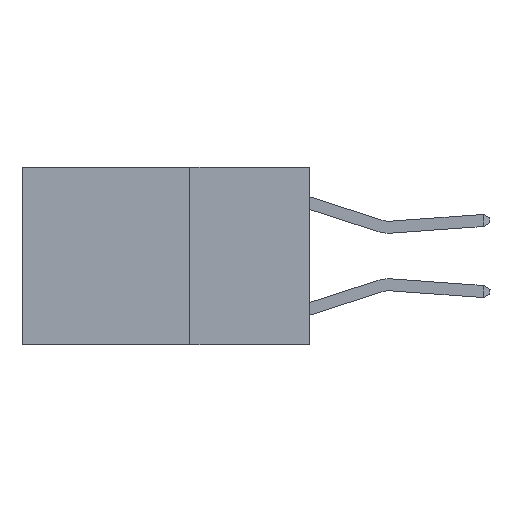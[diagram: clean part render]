
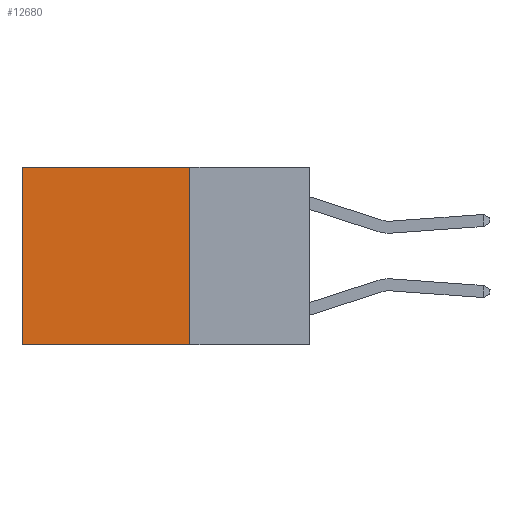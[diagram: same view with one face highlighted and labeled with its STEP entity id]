
A CAD part, left-side view. The second image highlights one B-rep face of the part: STEP entity #12680.
In plain terms, the highlighted planar face has unit normal (-1, 0, 0).
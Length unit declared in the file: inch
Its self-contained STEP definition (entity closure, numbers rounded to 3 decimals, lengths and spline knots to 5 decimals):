
#851 = LINE ( 'NONE', #23204, #16633 ) ;
#1499 = LINE ( 'NONE', #9269, #6930 ) ;
#1567 = ORIENTED_EDGE ( 'NONE', *, *, #6776, .T. ) ;
#1886 = ORIENTED_EDGE ( 'NONE', *, *, #24794, .F. ) ;
#3127 = VERTEX_POINT ( 'NONE', #9824 ) ;
#4340 = LINE ( 'NONE', #23465, #25507 ) ;
#4386 = EDGE_LOOP ( 'NONE', ( #1567, #4631, #1886, #12244 ) ) ;
#4631 = ORIENTED_EDGE ( 'NONE', *, *, #9931, .F. ) ;
#5051 = DIRECTION ( 'NONE',  ( 0., 0., -1. ) ) ;
#6243 = VERTEX_POINT ( 'NONE', #25667 ) ;
#6776 = EDGE_CURVE ( 'NONE', #3127, #23421, #851, .T. ) ;
#6930 = VECTOR ( 'NONE', #25627, 39.37008 ) ;
#9120 = CARTESIAN_POINT ( 'NONE',  ( 0.2625, 0.25, 0. ) ) ;
#9269 = CARTESIAN_POINT ( 'NONE',  ( 0.2625, 0.25, -0.37 ) ) ;
#9277 = CARTESIAN_POINT ( 'NONE',  ( 0.2625, 0.25, 0. ) ) ;
#9824 = CARTESIAN_POINT ( 'NONE',  ( 0.2625, 0.6, 0. ) ) ;
#9931 = EDGE_CURVE ( 'NONE', #19159, #23421, #1499, .T. ) ;
#11525 = EDGE_CURVE ( 'NONE', #6243, #3127, #24166, .T. ) ;
#12244 = ORIENTED_EDGE ( 'NONE', *, *, #11525, .T. ) ;
#12680 = ADVANCED_FACE ( 'NONE', ( #21945 ), #15362, .F. ) ;
#13265 = DIRECTION ( 'NONE',  ( 0., 0., -1. ) ) ;
#14783 = CARTESIAN_POINT ( 'NONE',  ( 0.2625, 0.25, -0.37 ) ) ;
#15362 = PLANE ( 'NONE',  #20645 ) ;
#16633 = VECTOR ( 'NONE', #25216, 39.37008 ) ;
#17469 = DIRECTION ( 'NONE',  ( 1., 0., 0. ) ) ;
#18775 = VECTOR ( 'NONE', #19648, 39.37008 ) ;
#19159 = VERTEX_POINT ( 'NONE', #14783 ) ;
#19648 = DIRECTION ( 'NONE',  ( 0., 1., 0. ) ) ;
#20046 = CARTESIAN_POINT ( 'NONE',  ( 0.2625, 0.6, -0.37 ) ) ;
#20645 = AXIS2_PLACEMENT_3D ( 'NONE', #9120, #17469, #5051 ) ;
#21945 = FACE_OUTER_BOUND ( 'NONE', #4386, .T. ) ;
#23204 = CARTESIAN_POINT ( 'NONE',  ( 0.2625, 0.6, 0. ) ) ;
#23421 = VERTEX_POINT ( 'NONE', #20046 ) ;
#23465 = CARTESIAN_POINT ( 'NONE',  ( 0.2625, 0.25, 0. ) ) ;
#24166 = LINE ( 'NONE', #9277, #18775 ) ;
#24794 = EDGE_CURVE ( 'NONE', #6243, #19159, #4340, .T. ) ;
#25216 = DIRECTION ( 'NONE',  ( 0., 0., -1. ) ) ;
#25507 = VECTOR ( 'NONE', #13265, 39.37008 ) ;
#25627 = DIRECTION ( 'NONE',  ( 0., 1., 0. ) ) ;
#25667 = CARTESIAN_POINT ( 'NONE',  ( 0.2625, 0.25, 0. ) ) ;
